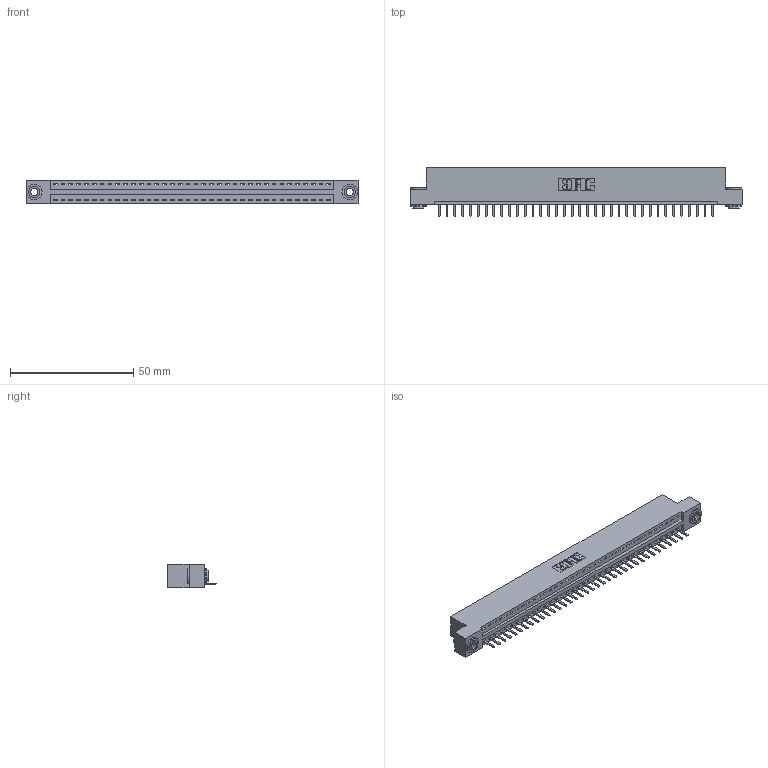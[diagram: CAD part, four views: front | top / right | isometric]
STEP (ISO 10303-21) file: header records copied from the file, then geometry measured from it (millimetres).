
FILE_DESCRIPTION (( 'STEP AP203' ), '1' );
FILE_NAME ('396-036-520-103.STEP', '2019-10-27T16:40:41', ( '' ), ( '' ), 'SwSTEP 2.0', 'SolidWorks 2016', '' );
FILE_SCHEMA (( 'CONFIG_CONTROL_DESIGN' ));
Length unit declared in the file: inch
Products named in the file (4): 345-292-001_345-293-120; 346 Part_Flush Mounting Lugs - 0.156 Dia-TH; 345-250-002_345-250-002-102; 396-036-520-103
Assembly tree (39 placements, depth 2):
  396-036-520-103
    346 Part_Flush Mounting Lugs - 0.156 Dia-TH
    345-292-001_345-293-120  x36
    345-250-002_345-250-002-102  x2
Bounding box: 134.87 x 20.02 x 9.4 mm (x, y, z)
Volume: 12784.9 mm3; surface area: 15788.3 mm2
Topology: 39 solids, 39 shells, 2392 faces, 7029 edges, 4586 vertices
Faces by surface type: plane 1598, cylinder 786, cone 8
Entity records: 23914 total; most frequent: CARTESIAN_POINT 4091, ORIENTED_EDGE 4042, DIRECTION 3635, EDGE_CURVE 2021, LINE 1717, VECTOR 1717, VERTEX_POINT 1342, AXIS2_PLACEMENT_3D 959
